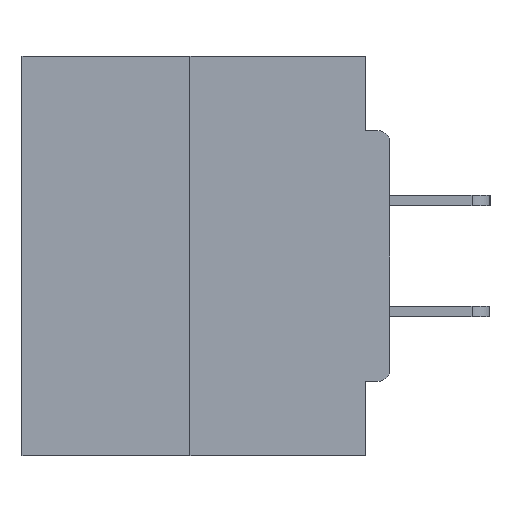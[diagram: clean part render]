
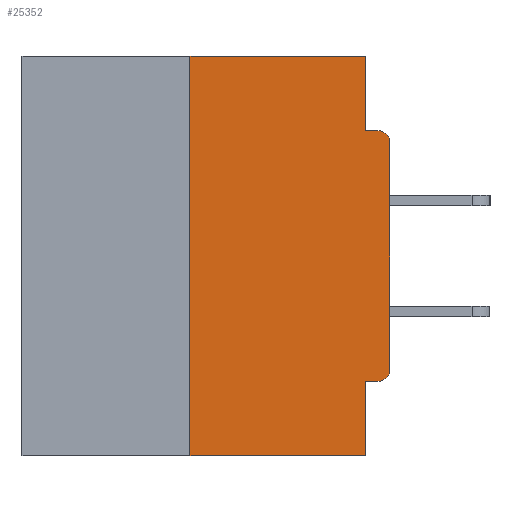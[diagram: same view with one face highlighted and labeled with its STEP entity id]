
A CAD part, left-side view. The second image highlights one B-rep face of the part: STEP entity #25352.
In plain terms, the highlighted planar face has unit normal (-1, 0, 0).
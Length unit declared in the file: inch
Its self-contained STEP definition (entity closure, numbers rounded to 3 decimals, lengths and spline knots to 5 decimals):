
#127 = DIRECTION ( 'NONE',  ( 1., 0., 0. ) ) ;
#635 = VECTOR ( 'NONE', #3747, 39.37008 ) ;
#751 = FACE_OUTER_BOUND ( 'NONE', #21795, .T. ) ;
#1095 = ORIENTED_EDGE ( 'NONE', *, *, #2756, .F. ) ;
#1312 = DIRECTION ( 'NONE',  ( 0., 1., 0. ) ) ;
#1865 = ORIENTED_EDGE ( 'NONE', *, *, #13021, .T. ) ;
#2407 = EDGE_CURVE ( 'NONE', #11658, #16693, #15745, .T. ) ;
#2756 = EDGE_CURVE ( 'NONE', #9604, #15014, #13669, .T. ) ;
#3747 = DIRECTION ( 'NONE',  ( 0., 0., -1. ) ) ;
#3907 = CARTESIAN_POINT ( 'NONE',  ( 0., 0.015, -0.4065 ) ) ;
#4771 = EDGE_CURVE ( 'NONE', #9577, #16693, #5793, .T. ) ;
#5366 = VERTEX_POINT ( 'NONE', #3907 ) ;
#5599 = CIRCLE ( 'NONE', #14197, 0.015 ) ;
#5793 = LINE ( 'NONE', #24561, #25758 ) ;
#6552 = CARTESIAN_POINT ( 'NONE',  ( 0., 0., -0.3915 ) ) ;
#7467 = VERTEX_POINT ( 'NONE', #24045 ) ;
#8184 = EDGE_CURVE ( 'NONE', #18999, #19461, #15288, .T. ) ;
#8388 = LINE ( 'NONE', #24665, #30021 ) ;
#9018 = DIRECTION ( 'NONE',  ( -1., 0., 0. ) ) ;
#9265 = ORIENTED_EDGE ( 'NONE', *, *, #32160, .T. ) ;
#9551 = VECTOR ( 'NONE', #24401, 39.37008 ) ;
#9577 = VERTEX_POINT ( 'NONE', #23626 ) ;
#9604 = VERTEX_POINT ( 'NONE', #19578 ) ;
#11658 = VERTEX_POINT ( 'NONE', #12705 ) ;
#11906 = ORIENTED_EDGE ( 'NONE', *, *, #4771, .F. ) ;
#12705 = CARTESIAN_POINT ( 'NONE',  ( 0., 0.25, -0.5 ) ) ;
#13021 = EDGE_CURVE ( 'NONE', #5366, #18999, #32181, .T. ) ;
#13669 = LINE ( 'NONE', #22397, #635 ) ;
#13852 = ORIENTED_EDGE ( 'NONE', *, *, #8184, .T. ) ;
#13868 = CARTESIAN_POINT ( 'NONE',  ( 0., 0., -0.0935 ) ) ;
#14197 = AXIS2_PLACEMENT_3D ( 'NONE', #24747, #9018, #27248 ) ;
#14289 = CARTESIAN_POINT ( 'NONE',  ( 0., 0., -0.4065 ) ) ;
#15014 = VERTEX_POINT ( 'NONE', #16922 ) ;
#15288 = LINE ( 'NONE', #18134, #16506 ) ;
#15507 = LINE ( 'NONE', #14289, #17948 ) ;
#15569 = ORIENTED_EDGE ( 'NONE', *, *, #32678, .F. ) ;
#15745 = LINE ( 'NONE', #20822, #28787 ) ;
#15792 = CARTESIAN_POINT ( 'NONE',  ( 0., 0.015, -0.0935 ) ) ;
#16053 = DIRECTION ( 'NONE',  ( 0., -1., 0. ) ) ;
#16444 = CARTESIAN_POINT ( 'NONE',  ( 0., 0.25, 0. ) ) ;
#16506 = VECTOR ( 'NONE', #25780, 39.37008 ) ;
#16693 = VERTEX_POINT ( 'NONE', #18392 ) ;
#16922 = CARTESIAN_POINT ( 'NONE',  ( 0., 0.031, -0.0935 ) ) ;
#17948 = VECTOR ( 'NONE', #1312, 39.37008 ) ;
#18134 = CARTESIAN_POINT ( 'NONE',  ( 0., 0., 0. ) ) ;
#18137 = CARTESIAN_POINT ( 'NONE',  ( 0., 0.46, 0. ) ) ;
#18392 = CARTESIAN_POINT ( 'NONE',  ( 0., 0.031, -0.5 ) ) ;
#18999 = VERTEX_POINT ( 'NONE', #6552 ) ;
#19141 = CARTESIAN_POINT ( 'NONE',  ( 0., 0.015, -0.3915 ) ) ;
#19461 = VERTEX_POINT ( 'NONE', #31505 ) ;
#19578 = CARTESIAN_POINT ( 'NONE',  ( 0., 0.031, 0. ) ) ;
#20028 = AXIS2_PLACEMENT_3D ( 'NONE', #18137, #127, #31050 ) ;
#20073 = VERTEX_POINT ( 'NONE', #15792 ) ;
#20653 = EDGE_CURVE ( 'NONE', #7467, #9604, #8388, .T. ) ;
#20822 = CARTESIAN_POINT ( 'NONE',  ( 0., 0.46, -0.5 ) ) ;
#21795 = EDGE_LOOP ( 'NONE', ( #30421, #30793, #33166, #11906, #15569, #1865, #13852, #9265, #28659, #1095 ) ) ;
#22397 = CARTESIAN_POINT ( 'NONE',  ( 0., 0.031, 0. ) ) ;
#23626 = CARTESIAN_POINT ( 'NONE',  ( 0., 0.031, -0.4065 ) ) ;
#24045 = CARTESIAN_POINT ( 'NONE',  ( 0., 0.25, 0. ) ) ;
#24401 = DIRECTION ( 'NONE',  ( 0., 0., 1. ) ) ;
#24561 = CARTESIAN_POINT ( 'NONE',  ( 0., 0.031, -0.5 ) ) ;
#24665 = CARTESIAN_POINT ( 'NONE',  ( 0., 0.46, 0. ) ) ;
#24725 = EDGE_CURVE ( 'NONE', #15014, #20073, #33060, .T. ) ;
#24747 = CARTESIAN_POINT ( 'NONE',  ( 0., 0.015, -0.1085 ) ) ;
#25352 = ADVANCED_FACE ( 'NONE', ( #751 ), #28622, .F. ) ;
#25719 = EDGE_CURVE ( 'NONE', #11658, #7467, #33677, .T. ) ;
#25758 = VECTOR ( 'NONE', #32253, 39.37008 ) ;
#25780 = DIRECTION ( 'NONE',  ( 0., 0., 1. ) ) ;
#27248 = DIRECTION ( 'NONE',  ( 0., 0., -1. ) ) ;
#27311 = VECTOR ( 'NONE', #16053, 39.37008 ) ;
#28622 = PLANE ( 'NONE',  #20028 ) ;
#28659 = ORIENTED_EDGE ( 'NONE', *, *, #24725, .F. ) ;
#28787 = VECTOR ( 'NONE', #28926, 39.37008 ) ;
#28926 = DIRECTION ( 'NONE',  ( 0., -1., 0. ) ) ;
#29392 = DIRECTION ( 'NONE',  ( 0., 0., -1. ) ) ;
#30021 = VECTOR ( 'NONE', #32709, 39.37008 ) ;
#30421 = ORIENTED_EDGE ( 'NONE', *, *, #20653, .F. ) ;
#30699 = AXIS2_PLACEMENT_3D ( 'NONE', #19141, #32316, #29392 ) ;
#30793 = ORIENTED_EDGE ( 'NONE', *, *, #25719, .F. ) ;
#31050 = DIRECTION ( 'NONE',  ( 0., 0., -1. ) ) ;
#31505 = CARTESIAN_POINT ( 'NONE',  ( 0., 0., -0.1085 ) ) ;
#32160 = EDGE_CURVE ( 'NONE', #19461, #20073, #5599, .T. ) ;
#32181 = CIRCLE ( 'NONE', #30699, 0.015 ) ;
#32253 = DIRECTION ( 'NONE',  ( 0., 0., -1. ) ) ;
#32316 = DIRECTION ( 'NONE',  ( -1., 0., 0. ) ) ;
#32678 = EDGE_CURVE ( 'NONE', #5366, #9577, #15507, .T. ) ;
#32709 = DIRECTION ( 'NONE',  ( 0., -1., 0. ) ) ;
#33060 = LINE ( 'NONE', #13868, #27311 ) ;
#33166 = ORIENTED_EDGE ( 'NONE', *, *, #2407, .T. ) ;
#33677 = LINE ( 'NONE', #16444, #9551 ) ;
